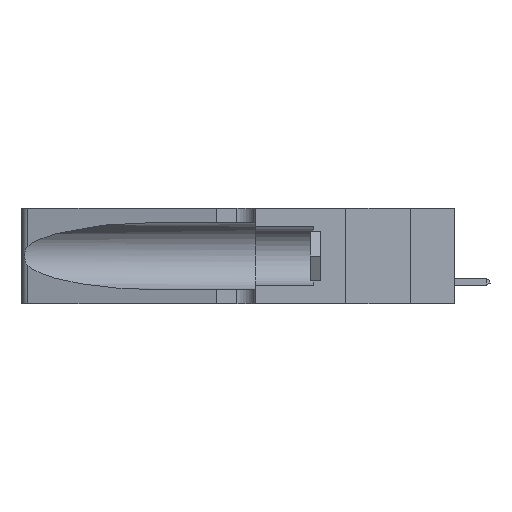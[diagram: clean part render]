
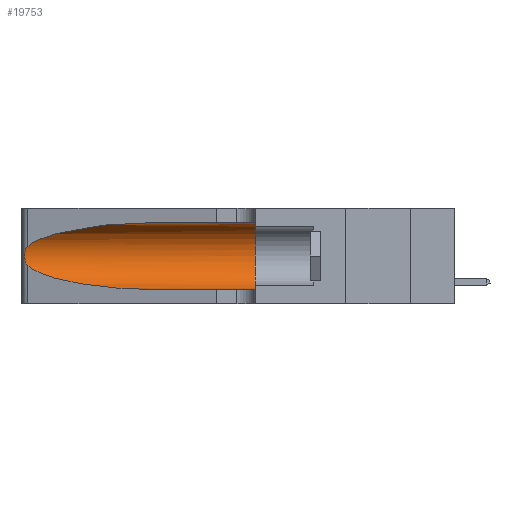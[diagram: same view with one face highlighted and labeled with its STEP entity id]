
A CAD part, left-side view. The second image highlights one B-rep face of the part: STEP entity #19753.
In plain terms, the highlighted cylindrical face has radius 3.308 mm (diameter 6.617 mm), a partial arc.
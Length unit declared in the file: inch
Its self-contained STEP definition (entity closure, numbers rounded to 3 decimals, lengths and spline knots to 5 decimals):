
#1093 = CARTESIAN_POINT ( 'NONE',  ( 0.1305, 1.61858, 0.185 ) ) ;
#1117 = CARTESIAN_POINT ( 'NONE',  ( 0.25639, 1.23184, 0.21858 ) ) ;
#1419 = CARTESIAN_POINT ( 'NONE',  ( 0.25854, 1.2359, 0.20912 ) ) ;
#1502 = CARTESIAN_POINT ( 'NONE',  ( 0.2373, 1.15595, 0.08982 ) ) ;
#1642 = CYLINDRICAL_SURFACE ( 'NONE', #10784, 0.13025 ) ;
#1734 = CARTESIAN_POINT ( 'NONE',  ( 0.25856, 1.23593, 0.16098 ) ) ;
#1813 = CARTESIAN_POINT ( 'NONE',  ( 0.26018, 1.23835, 0.19895 ) ) ;
#2474 = FACE_OUTER_BOUND ( 'NONE', #17054, .T. ) ;
#2531 = CARTESIAN_POINT ( 'NONE',  ( 0.25487, 1.22718, 0.22369 ) ) ;
#2764 =( BOUNDED_CURVE ( )  B_SPLINE_CURVE ( 3, ( #18298, #18143, #3546, #21778 ),
 .UNSPECIFIED., .F., .T. ) 
 B_SPLINE_CURVE_WITH_KNOTS ( ( 4, 4 ),
 ( 1.5708, 2.84003 ),
 .UNSPECIFIED. ) 
 CURVE ( )  GEOMETRIC_REPRESENTATION_ITEM ( )  RATIONAL_B_SPLINE_CURVE ( ( 1., 0.87, 0.87, 1. ) ) 
 REPRESENTATION_ITEM ( '' )  );
#3114 = CARTESIAN_POINT ( 'NONE',  ( 0.1305, 0.35, 0.185 ) ) ;
#3197 = ORIENTED_EDGE ( 'NONE', *, *, #20956, .T. ) ;
#3373 = CARTESIAN_POINT ( 'NONE',  ( 0.26075, 1.23896, 0.178 ) ) ;
#3546 = CARTESIAN_POINT ( 'NONE',  ( 0.2373, 1.15595, 0.28018 ) ) ;
#3653 = B_SPLINE_CURVE_WITH_KNOTS ( 'NONE', 3,
 ( #2531, #6320, #1117, #20891, #1419, #1813, #23350, #3373, #8871, #1734, #15893, #10652, #15964, #5222 ),
 .UNSPECIFIED., .F., .F.,
 ( 4, 2, 2, 2, 2, 2, 4 ),
 ( 0., 0.00027, 0.00053, 0.00107, 0.0016, 0.00187, 0.00214 ),
 .UNSPECIFIED. ) ;
#4098 = CARTESIAN_POINT ( 'NONE',  ( 0.18966, 0.96281, 0.05475 ) ) ;
#4952 = DIRECTION ( 'NONE',  ( 0., 1., 0. ) ) ;
#5222 = CARTESIAN_POINT ( 'NONE',  ( 0.25487, 1.22718, 0.14631 ) ) ;
#5289 = VERTEX_POINT ( 'NONE', #20111 ) ;
#5754 = EDGE_CURVE ( 'NONE', #21907, #19368, #7687, .T. ) ;
#5940 = CARTESIAN_POINT ( 'NONE',  ( 0.1305, 0.72297, 0.05475 ) ) ;
#6220 = LINE ( 'NONE', #7491, #20039 ) ;
#6229 = EDGE_CURVE ( 'NONE', #23111, #18959, #6220, .T. ) ;
#6320 = CARTESIAN_POINT ( 'NONE',  ( 0.25555, 1.22994, 0.2215 ) ) ;
#6446 = DIRECTION ( 'NONE',  ( 0., -1., 0. ) ) ;
#6737 = VERTEX_POINT ( 'NONE', #10169 ) ;
#7491 = CARTESIAN_POINT ( 'NONE',  ( 0.1305, 1.61858, 0.31525 ) ) ;
#7687 = LINE ( 'NONE', #21067, #10505 ) ;
#7831 = CARTESIAN_POINT ( 'NONE',  ( 0.1305, 0.72297, 0.05475 ) ) ;
#8526 = DIRECTION ( 'NONE',  ( 0., 0., 1. ) ) ;
#8603 = DIRECTION ( 'NONE',  ( 0., 0., -1. ) ) ;
#8724 = CARTESIAN_POINT ( 'NONE',  ( 0.25487, 1.22718, 0.14631 ) ) ;
#8871 = CARTESIAN_POINT ( 'NONE',  ( 0.26017, 1.23833, 0.17102 ) ) ;
#9770 = ORIENTED_EDGE ( 'NONE', *, *, #6229, .F. ) ;
#10025 = EDGE_CURVE ( 'NONE', #6737, #5289, #3653, .T. ) ;
#10169 = CARTESIAN_POINT ( 'NONE',  ( 0.25487, 1.22718, 0.22369 ) ) ;
#10473 = ORIENTED_EDGE ( 'NONE', *, *, #10025, .T. ) ;
#10505 = VECTOR ( 'NONE', #12098, 39.37008 ) ;
#10562 = EDGE_CURVE ( 'NONE', #5289, #21907, #13195, .T. ) ;
#10652 = CARTESIAN_POINT ( 'NONE',  ( 0.25639, 1.23186, 0.15144 ) ) ;
#10784 = AXIS2_PLACEMENT_3D ( 'NONE', #1093, #15550, #8603 ) ;
#12098 = DIRECTION ( 'NONE',  ( 0., -1., 0. ) ) ;
#13055 = CARTESIAN_POINT ( 'NONE',  ( 0.1305, 0.35, 0.05475 ) ) ;
#13195 =( BOUNDED_CURVE ( )  B_SPLINE_CURVE ( 3, ( #8724, #1502, #4098, #7831 ),
 .UNSPECIFIED., .F., .T. ) 
 B_SPLINE_CURVE_WITH_KNOTS ( ( 4, 4 ),
 ( 3.44316, 4.71239 ),
 .UNSPECIFIED. ) 
 CURVE ( )  GEOMETRIC_REPRESENTATION_ITEM ( )  RATIONAL_B_SPLINE_CURVE ( ( 1., 0.87, 0.87, 1. ) ) 
 REPRESENTATION_ITEM ( '' )  );
#13386 = CARTESIAN_POINT ( 'NONE',  ( 0.1305, 0.35, 0.31525 ) ) ;
#14991 = CIRCLE ( 'NONE', #19060, 0.13025 ) ;
#15550 = DIRECTION ( 'NONE',  ( 0., -1., 0. ) ) ;
#15893 = CARTESIAN_POINT ( 'NONE',  ( 0.25789, 1.23486, 0.15765 ) ) ;
#15964 = CARTESIAN_POINT ( 'NONE',  ( 0.25555, 1.22993, 0.14849 ) ) ;
#16053 = ORIENTED_EDGE ( 'NONE', *, *, #5754, .T. ) ;
#17054 = EDGE_LOOP ( 'NONE', ( #3197, #10473, #18856, #16053, #18091, #9770 ) ) ;
#18053 = EDGE_CURVE ( 'NONE', #18959, #19368, #14991, .T. ) ;
#18091 = ORIENTED_EDGE ( 'NONE', *, *, #18053, .F. ) ;
#18143 = CARTESIAN_POINT ( 'NONE',  ( 0.18966, 0.96281, 0.31525 ) ) ;
#18254 = CARTESIAN_POINT ( 'NONE',  ( 0.1305, 0.72297, 0.31525 ) ) ;
#18298 = CARTESIAN_POINT ( 'NONE',  ( 0.1305, 0.72297, 0.31525 ) ) ;
#18856 = ORIENTED_EDGE ( 'NONE', *, *, #10562, .T. ) ;
#18959 = VERTEX_POINT ( 'NONE', #13386 ) ;
#19060 = AXIS2_PLACEMENT_3D ( 'NONE', #3114, #4952, #8526 ) ;
#19368 = VERTEX_POINT ( 'NONE', #13055 ) ;
#19753 = ADVANCED_FACE ( 'NONE', ( #2474 ), #1642, .F. ) ;
#20039 = VECTOR ( 'NONE', #6446, 39.37008 ) ;
#20111 = CARTESIAN_POINT ( 'NONE',  ( 0.25487, 1.22718, 0.14631 ) ) ;
#20891 = CARTESIAN_POINT ( 'NONE',  ( 0.25787, 1.23484, 0.2124 ) ) ;
#20956 = EDGE_CURVE ( 'NONE', #23111, #6737, #2764, .T. ) ;
#21067 = CARTESIAN_POINT ( 'NONE',  ( 0.1305, 1.61858, 0.05475 ) ) ;
#21778 = CARTESIAN_POINT ( 'NONE',  ( 0.25487, 1.22718, 0.22369 ) ) ;
#21907 = VERTEX_POINT ( 'NONE', #5940 ) ;
#23111 = VERTEX_POINT ( 'NONE', #18254 ) ;
#23350 = CARTESIAN_POINT ( 'NONE',  ( 0.26075, 1.23896, 0.19203 ) ) ;
